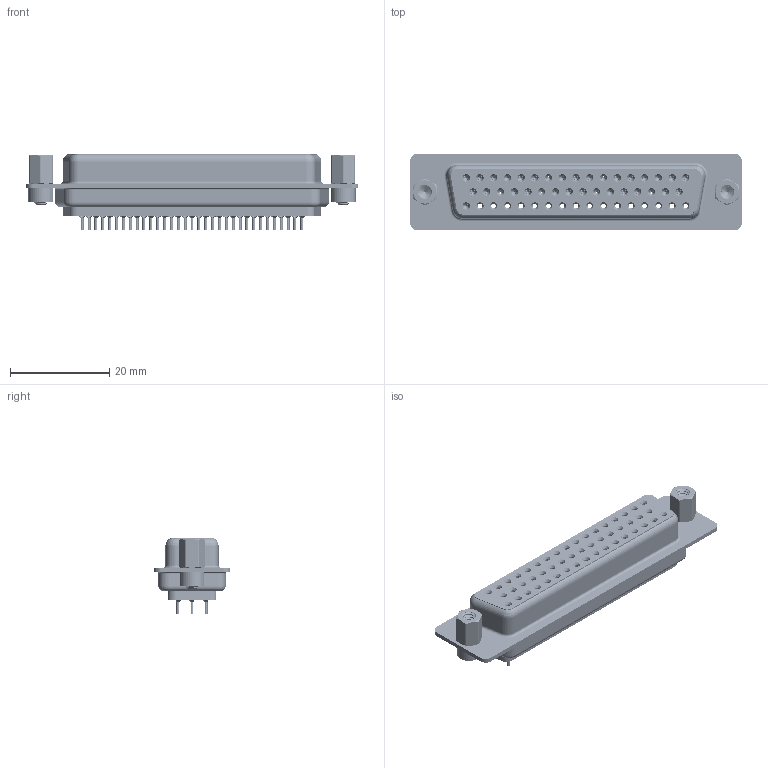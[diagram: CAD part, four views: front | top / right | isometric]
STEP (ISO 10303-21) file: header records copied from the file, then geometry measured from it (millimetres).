
FILE_DESCRIPTION (( 'STEP AP203' ), '1' );
FILE_NAME ('628-050-228-543.STEP', '2018-10-20T09:01:38', ( '' ), ( '' ), 'SwSTEP 2.0', 'SolidWorks 2016', '' );
FILE_SCHEMA (( 'CONFIG_CONTROL_DESIGN' ));
Length unit declared in the file: millimetre
Products named in the file (9): 628 Contact Row 2_28L; 628 Contact Row 3_28L; 628 4-40 Threaded Rivet; 628 4-40 Hex Standoff; 628-050-228-543; 628 Housing_50 LP; 628 Shell Front_50 Contacts; 628 Shell Rear_50 Contacts; 628 Contact Row 1_28L
Assembly tree (41 placements, depth 2):
  628-050-228-543
    628 Housing_50 LP
    628 Shell Front_50 Contacts
    628 Shell Rear_50 Contacts
    628 Contact Row 1_28L  x17
    628 Contact Row 2_28L  x16
    628 Contact Row 3_28L
    628 4-40 Threaded Rivet  x2
    628 4-40 Hex Standoff  x2
Bounding box: 67 x 15.4 x 15.3 mm (x, y, z)
Volume: 6794.6 mm3; surface area: 14084.9 mm2
Topology: 41 solids, 41 shells, 4931 faces, 12499 edges, 7777 vertices
Faces by surface type: cylinder 1459, plane 1191, torus 947, bspline 698, cone 636
Entity records: 46542 total; most frequent: CARTESIAN_POINT 14454, DIRECTION 6652, ORIENTED_EDGE 6100, EDGE_CURVE 3050, AXIS2_PLACEMENT_3D 2799, VERTEX_POINT 1932, EDGE_LOOP 1570, CIRCLE 1529
